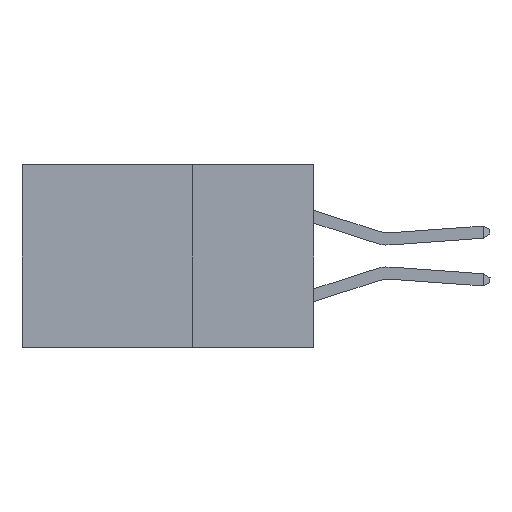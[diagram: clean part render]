
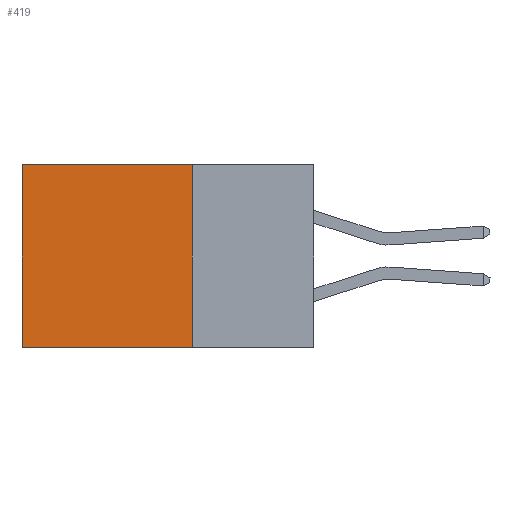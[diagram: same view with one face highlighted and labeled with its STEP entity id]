
A CAD part, left-side view. The second image highlights one B-rep face of the part: STEP entity #419.
In plain terms, the highlighted planar face has unit normal (-1, 0, 0).
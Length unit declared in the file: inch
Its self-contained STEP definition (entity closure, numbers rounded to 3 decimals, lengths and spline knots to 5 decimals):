
#72 = CARTESIAN_POINT ( 'NONE',  ( 0.2875, 0.25, 0. ) ) ;
#419 = ADVANCED_FACE ( 'NONE', ( #16879 ), #17965, .F. ) ;
#751 = VERTEX_POINT ( 'NONE', #21640 ) ;
#807 = VECTOR ( 'NONE', #10681, 39.37008 ) ;
#2617 = ORIENTED_EDGE ( 'NONE', *, *, #22976, .T. ) ;
#2749 = EDGE_CURVE ( 'NONE', #8740, #19989, #17865, .T. ) ;
#2783 = LINE ( 'NONE', #72, #807 ) ;
#2886 = ORIENTED_EDGE ( 'NONE', *, *, #5307, .F. ) ;
#3357 = EDGE_CURVE ( 'NONE', #751, #17338, #2783, .T. ) ;
#4285 = LINE ( 'NONE', #20734, #13237 ) ;
#4833 = CARTESIAN_POINT ( 'NONE',  ( 0.2875, 0.25, -0.375 ) ) ;
#5307 = EDGE_CURVE ( 'NONE', #751, #8740, #15302, .T. ) ;
#6461 = DIRECTION ( 'NONE',  ( 0., 0., -1. ) ) ;
#6477 = CARTESIAN_POINT ( 'NONE',  ( 0.2875, 0.25, -0.375 ) ) ;
#7132 = DIRECTION ( 'NONE',  ( 1., 0., 0. ) ) ;
#7293 = CARTESIAN_POINT ( 'NONE',  ( 0.2875, 0.25, -0.375 ) ) ;
#7575 = CARTESIAN_POINT ( 'NONE',  ( 0.2875, 0.6, 0. ) ) ;
#8740 = VERTEX_POINT ( 'NONE', #10860 ) ;
#9996 = ORIENTED_EDGE ( 'NONE', *, *, #2749, .F. ) ;
#10084 = VECTOR ( 'NONE', #17024, 39.37008 ) ;
#10681 = DIRECTION ( 'NONE',  ( 0., 1., 0. ) ) ;
#10860 = CARTESIAN_POINT ( 'NONE',  ( 0.2875, 0.25, -0.375 ) ) ;
#11096 = VECTOR ( 'NONE', #6461, 39.37008 ) ;
#11805 = EDGE_LOOP ( 'NONE', ( #2617, #9996, #2886, #13290 ) ) ;
#13237 = VECTOR ( 'NONE', #22519, 39.37008 ) ;
#13290 = ORIENTED_EDGE ( 'NONE', *, *, #3357, .T. ) ;
#13608 = AXIS2_PLACEMENT_3D ( 'NONE', #7293, #7132, #16269 ) ;
#15302 = LINE ( 'NONE', #4833, #11096 ) ;
#16269 = DIRECTION ( 'NONE',  ( 0., 0., -1. ) ) ;
#16655 = CARTESIAN_POINT ( 'NONE',  ( 0.2875, 0.6, -0.375 ) ) ;
#16879 = FACE_OUTER_BOUND ( 'NONE', #11805, .T. ) ;
#17024 = DIRECTION ( 'NONE',  ( 0., 1., 0. ) ) ;
#17338 = VERTEX_POINT ( 'NONE', #7575 ) ;
#17865 = LINE ( 'NONE', #6477, #10084 ) ;
#17965 = PLANE ( 'NONE',  #13608 ) ;
#19989 = VERTEX_POINT ( 'NONE', #16655 ) ;
#20734 = CARTESIAN_POINT ( 'NONE',  ( 0.2875, 0.6, -0.375 ) ) ;
#21640 = CARTESIAN_POINT ( 'NONE',  ( 0.2875, 0.25, 0. ) ) ;
#22519 = DIRECTION ( 'NONE',  ( 0., 0., -1. ) ) ;
#22976 = EDGE_CURVE ( 'NONE', #17338, #19989, #4285, .T. ) ;
